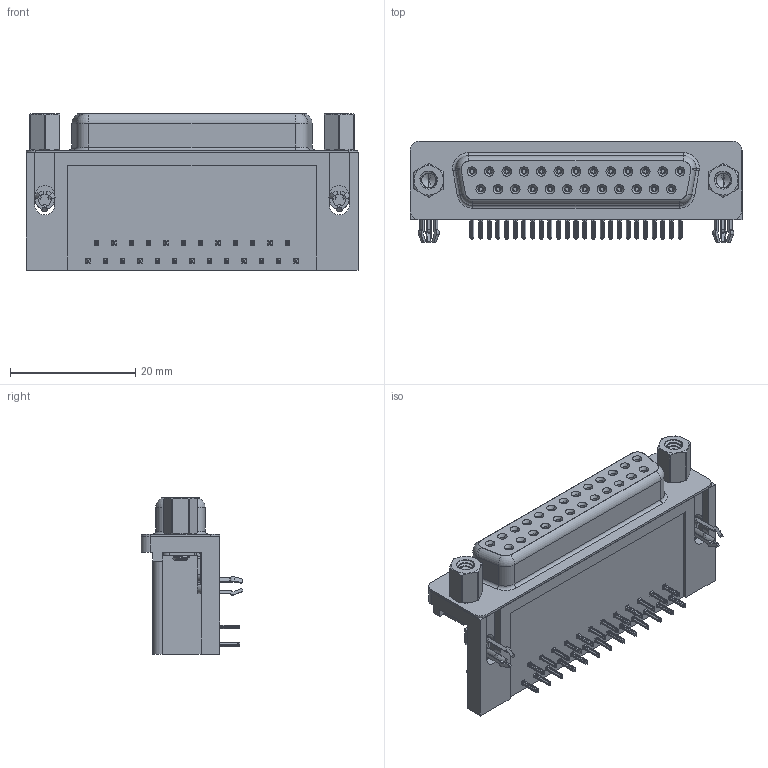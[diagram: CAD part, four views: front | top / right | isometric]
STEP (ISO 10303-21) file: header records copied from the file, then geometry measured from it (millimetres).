
FILE_DESCRIPTION (( 'STEP AP203' ), '1' );
FILE_NAME ('626-025-262-042.STEP', '2018-11-07T02:32:24', ( '' ), ( '' ), 'SwSTEP 2.0', 'SolidWorks 2016', '' );
FILE_SCHEMA (( 'CONFIG_CONTROL_DESIGN' ));
Length unit declared in the file: millimetre
Products named in the file (7): 626 Contact Bottom; 626 Contact Top; 626 3 Prong Board Lock; 626 4-40 Hex Standoff 5; 626-025-262-042; 626 Housing_25 Socket; 626 Shell_25 Socket
Assembly tree (31 placements, depth 2):
  626-025-262-042
    626 Housing_25 Socket
    626 Shell_25 Socket
    626 Contact Bottom  x12
    626 Contact Top  x13
    626 3 Prong Board Lock  x2
    626 4-40 Hex Standoff 5  x2
Bounding box: 53.04 x 16.25 x 24.96 mm (x, y, z)
Volume: 10810.1 mm3; surface area: 11587.7 mm2
Topology: 31 solids, 31 shells, 3992 faces, 10540 edges, 6626 vertices
Faces by surface type: plane 1766, cylinder 960, bspline 864, cone 356, torus 46
Entity records: 34333 total; most frequent: CARTESIAN_POINT 11274, ORIENTED_EDGE 4644, DIRECTION 4235, EDGE_CURVE 2322, VERTEX_POINT 1489, VECTOR 1459, LINE 1459, AXIS2_PLACEMENT_3D 1388
